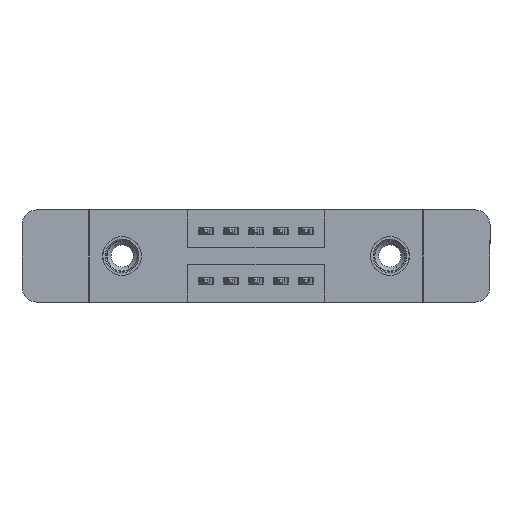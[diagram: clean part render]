
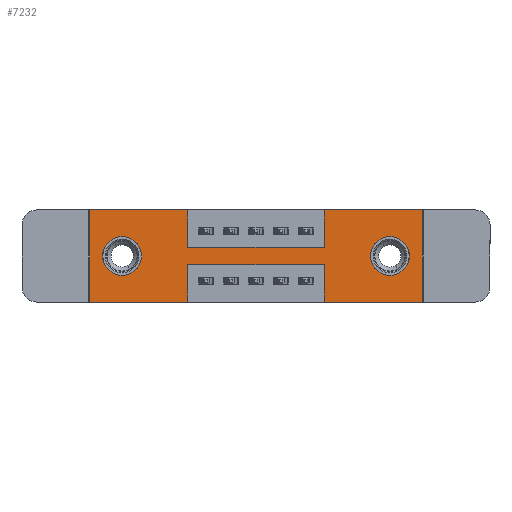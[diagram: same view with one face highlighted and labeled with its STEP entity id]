
A CAD part, front view. The second image highlights one B-rep face of the part: STEP entity #7232.
In plain terms, the highlighted planar face has unit normal (0, -1, 0).
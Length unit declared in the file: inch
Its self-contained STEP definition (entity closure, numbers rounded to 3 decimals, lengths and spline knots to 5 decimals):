
#77 = VERTEX_POINT ( 'NONE', #6850 ) ;
#149 = VECTOR ( 'NONE', #7462, 39.37008 ) ;
#326 = EDGE_CURVE ( 'NONE', #3214, #6701, #7001, .T. ) ;
#468 = DIRECTION ( 'NONE',  ( 0., -1., 0. ) ) ;
#501 = ORIENTED_EDGE ( 'NONE', *, *, #8408, .F. ) ;
#829 = EDGE_LOOP ( 'NONE', ( #4135, #11269 ) ) ;
#876 = DIRECTION ( 'NONE',  ( 0., 0., -1. ) ) ;
#897 = VECTOR ( 'NONE', #2750, 39.37008 ) ;
#1196 = VERTEX_POINT ( 'NONE', #5512 ) ;
#1234 = DIRECTION ( 'NONE',  ( 0., 1., 0. ) ) ;
#1258 = VERTEX_POINT ( 'NONE', #2331 ) ;
#1437 = CARTESIAN_POINT ( 'NONE',  ( 0., 0., -0.37 ) ) ;
#1601 = CARTESIAN_POINT ( 'NONE',  ( 0.13, 0., -0.185 ) ) ;
#1706 = FACE_OUTER_BOUND ( 'NONE', #3340, .T. ) ;
#1759 = DIRECTION ( 'NONE',  ( 0., 0., 1. ) ) ;
#1939 = EDGE_CURVE ( 'NONE', #1196, #9903, #5960, .T. ) ;
#2300 = CIRCLE ( 'NONE', #10257, 0.078 ) ;
#2305 = VERTEX_POINT ( 'NONE', #12155 ) ;
#2312 = CARTESIAN_POINT ( 'NONE',  ( 0.9425, 0., 0. ) ) ;
#2331 = CARTESIAN_POINT ( 'NONE',  ( 0.9425, 0., -0.37 ) ) ;
#2378 = FACE_BOUND ( 'NONE', #8238, .T. ) ;
#2586 = LINE ( 'NONE', #11215, #7533 ) ;
#2589 = CARTESIAN_POINT ( 'NONE',  ( 0., 0., -0.37 ) ) ;
#2598 = ORIENTED_EDGE ( 'NONE', *, *, #13503, .T. ) ;
#2750 = DIRECTION ( 'NONE',  ( 0., 0., -1. ) ) ;
#2804 = LINE ( 'NONE', #5063, #12337 ) ;
#3098 = DIRECTION ( 'NONE',  ( 1., 0., 0. ) ) ;
#3123 = CARTESIAN_POINT ( 'NONE',  ( 0., 0., -0.37 ) ) ;
#3214 = VERTEX_POINT ( 'NONE', #5494 ) ;
#3245 = CARTESIAN_POINT ( 'NONE',  ( 0., 0., 0. ) ) ;
#3257 = AXIS2_PLACEMENT_3D ( 'NONE', #12793, #12705, #6211 ) ;
#3306 = CARTESIAN_POINT ( 'NONE',  ( 1.205, 0., -0.107 ) ) ;
#3326 = VERTEX_POINT ( 'NONE', #8936 ) ;
#3340 = EDGE_LOOP ( 'NONE', ( #4166, #6298, #8539, #12453, #501, #4323, #7828, #5937, #9986, #5646, #8807, #5142 ) ) ;
#3584 = CARTESIAN_POINT ( 'NONE',  ( 0.9425, 0., -0.37 ) ) ;
#3618 = DIRECTION ( 'NONE',  ( 0., 0., -1. ) ) ;
#3710 = PLANE ( 'NONE',  #12693 ) ;
#3730 = CARTESIAN_POINT ( 'NONE',  ( 0.3925, 0., 0. ) ) ;
#3761 = EDGE_CURVE ( 'NONE', #3326, #12559, #2804, .T. ) ;
#3765 = DIRECTION ( 'NONE',  ( 0., 0., -1. ) ) ;
#3780 = LINE ( 'NONE', #6078, #897 ) ;
#3828 = EDGE_CURVE ( 'NONE', #6957, #2305, #9425, .T. ) ;
#4032 = VERTEX_POINT ( 'NONE', #4466 ) ;
#4135 = ORIENTED_EDGE ( 'NONE', *, *, #3828, .T. ) ;
#4166 = ORIENTED_EDGE ( 'NONE', *, *, #5066, .F. ) ;
#4209 = EDGE_CURVE ( 'NONE', #13288, #11241, #8897, .T. ) ;
#4323 = ORIENTED_EDGE ( 'NONE', *, *, #326, .F. ) ;
#4449 = CARTESIAN_POINT ( 'NONE',  ( 0.13, 0., -0.107 ) ) ;
#4466 = CARTESIAN_POINT ( 'NONE',  ( 0.3925, 0., -0.15 ) ) ;
#4483 = EDGE_CURVE ( 'NONE', #6634, #6899, #14109, .T. ) ;
#4513 = CARTESIAN_POINT ( 'NONE',  ( 0., 0., 0. ) ) ;
#4655 = LINE ( 'NONE', #3730, #5844 ) ;
#4662 = DIRECTION ( 'NONE',  ( 0., 0., 1. ) ) ;
#4938 = LINE ( 'NONE', #2312, #9140 ) ;
#4954 = LINE ( 'NONE', #3123, #149 ) ;
#5063 = CARTESIAN_POINT ( 'NONE',  ( 0.3925, 0., -0.22 ) ) ;
#5066 = EDGE_CURVE ( 'NONE', #12559, #13288, #3780, .T. ) ;
#5142 = ORIENTED_EDGE ( 'NONE', *, *, #4209, .F. ) ;
#5155 = VECTOR ( 'NONE', #6878, 39.37008 ) ;
#5494 = CARTESIAN_POINT ( 'NONE',  ( 0.9425, 0., 0. ) ) ;
#5512 = CARTESIAN_POINT ( 'NONE',  ( 1.205, 0., -0.263 ) ) ;
#5526 = CARTESIAN_POINT ( 'NONE',  ( 0., 0., 0. ) ) ;
#5646 = ORIENTED_EDGE ( 'NONE', *, *, #4483, .F. ) ;
#5674 = DIRECTION ( 'NONE',  ( 0., 0., 1. ) ) ;
#5718 = EDGE_CURVE ( 'NONE', #6899, #4032, #4655, .T. ) ;
#5844 = VECTOR ( 'NONE', #876, 39.37008 ) ;
#5937 = ORIENTED_EDGE ( 'NONE', *, *, #6032, .F. ) ;
#5960 = CIRCLE ( 'NONE', #3257, 0.078 ) ;
#6032 = EDGE_CURVE ( 'NONE', #4032, #77, #2586, .T. ) ;
#6078 = CARTESIAN_POINT ( 'NONE',  ( 0.3925, 0., -0.37 ) ) ;
#6211 = DIRECTION ( 'NONE',  ( 0., 0., -1. ) ) ;
#6298 = ORIENTED_EDGE ( 'NONE', *, *, #3761, .F. ) ;
#6305 = CARTESIAN_POINT ( 'NONE',  ( 1.335, 0., -0.37 ) ) ;
#6488 = CARTESIAN_POINT ( 'NONE',  ( 0., 0., 0. ) ) ;
#6634 = VERTEX_POINT ( 'NONE', #4513 ) ;
#6701 = VERTEX_POINT ( 'NONE', #9214 ) ;
#6850 = CARTESIAN_POINT ( 'NONE',  ( 0.9425, 0., -0.15 ) ) ;
#6862 = DIRECTION ( 'NONE',  ( 0., 1., 0. ) ) ;
#6878 = DIRECTION ( 'NONE',  ( 0., 0., 1. ) ) ;
#6899 = VERTEX_POINT ( 'NONE', #10022 ) ;
#6928 = EDGE_CURVE ( 'NONE', #1258, #3326, #7993, .T. ) ;
#6933 = DIRECTION ( 'NONE',  ( 0., 1., 0. ) ) ;
#6957 = VERTEX_POINT ( 'NONE', #4449 ) ;
#7001 = LINE ( 'NONE', #6488, #12428 ) ;
#7232 = ADVANCED_FACE ( 'NONE', ( #2378, #13116, #1706 ), #3710, .T. ) ;
#7245 = DIRECTION ( 'NONE',  ( -1., 0., 0. ) ) ;
#7459 = EDGE_CURVE ( 'NONE', #9203, #1258, #4954, .T. ) ;
#7462 = DIRECTION ( 'NONE',  ( -1., 0., 0. ) ) ;
#7533 = VECTOR ( 'NONE', #9066, 39.37008 ) ;
#7828 = ORIENTED_EDGE ( 'NONE', *, *, #7891, .F. ) ;
#7891 = EDGE_CURVE ( 'NONE', #77, #3214, #4938, .T. ) ;
#7902 = CARTESIAN_POINT ( 'NONE',  ( 1.335, 0., 0. ) ) ;
#7993 = LINE ( 'NONE', #3584, #5155 ) ;
#8165 = CARTESIAN_POINT ( 'NONE',  ( 0.3925, 0., -0.22 ) ) ;
#8202 = EDGE_CURVE ( 'NONE', #11241, #6634, #10683, .T. ) ;
#8215 = CARTESIAN_POINT ( 'NONE',  ( 0., 0., -0.37 ) ) ;
#8238 = EDGE_LOOP ( 'NONE', ( #2598, #11812 ) ) ;
#8408 = EDGE_CURVE ( 'NONE', #6701, #9203, #11704, .T. ) ;
#8441 = AXIS2_PLACEMENT_3D ( 'NONE', #12156, #1234, #11009 ) ;
#8539 = ORIENTED_EDGE ( 'NONE', *, *, #6928, .F. ) ;
#8807 = ORIENTED_EDGE ( 'NONE', *, *, #8202, .F. ) ;
#8897 = LINE ( 'NONE', #8215, #10082 ) ;
#8936 = CARTESIAN_POINT ( 'NONE',  ( 0.9425, 0., -0.22 ) ) ;
#9066 = DIRECTION ( 'NONE',  ( 1., 0., 0. ) ) ;
#9140 = VECTOR ( 'NONE', #5674, 39.37008 ) ;
#9203 = VERTEX_POINT ( 'NONE', #6305 ) ;
#9214 = CARTESIAN_POINT ( 'NONE',  ( 1.335, 0., 0. ) ) ;
#9274 = DIRECTION ( 'NONE',  ( -1., 0., 0. ) ) ;
#9425 = CIRCLE ( 'NONE', #11366, 0.078 ) ;
#9903 = VERTEX_POINT ( 'NONE', #3306 ) ;
#9986 = ORIENTED_EDGE ( 'NONE', *, *, #5718, .F. ) ;
#10022 = CARTESIAN_POINT ( 'NONE',  ( 0.3925, 0., 0. ) ) ;
#10082 = VECTOR ( 'NONE', #7245, 39.37008 ) ;
#10257 = AXIS2_PLACEMENT_3D ( 'NONE', #1601, #6933, #4662 ) ;
#10312 = VECTOR ( 'NONE', #3098, 39.37008 ) ;
#10516 = VECTOR ( 'NONE', #13121, 39.37008 ) ;
#10683 = LINE ( 'NONE', #5526, #10516 ) ;
#10812 = DIRECTION ( 'NONE',  ( 1., 0., 0. ) ) ;
#11009 = DIRECTION ( 'NONE',  ( 0., 0., -1. ) ) ;
#11215 = CARTESIAN_POINT ( 'NONE',  ( 0.3925, 0., -0.15 ) ) ;
#11241 = VERTEX_POINT ( 'NONE', #2589 ) ;
#11269 = ORIENTED_EDGE ( 'NONE', *, *, #14064, .T. ) ;
#11366 = AXIS2_PLACEMENT_3D ( 'NONE', #13342, #6862, #1759 ) ;
#11704 = LINE ( 'NONE', #7902, #13422 ) ;
#11792 = CARTESIAN_POINT ( 'NONE',  ( 0.3925, 0., -0.37 ) ) ;
#11812 = ORIENTED_EDGE ( 'NONE', *, *, #1939, .T. ) ;
#11831 = CIRCLE ( 'NONE', #8441, 0.078 ) ;
#12155 = CARTESIAN_POINT ( 'NONE',  ( 0.13, 0., -0.263 ) ) ;
#12156 = CARTESIAN_POINT ( 'NONE',  ( 1.205, 0., -0.185 ) ) ;
#12337 = VECTOR ( 'NONE', #9274, 39.37008 ) ;
#12428 = VECTOR ( 'NONE', #10812, 39.37008 ) ;
#12453 = ORIENTED_EDGE ( 'NONE', *, *, #7459, .F. ) ;
#12559 = VERTEX_POINT ( 'NONE', #8165 ) ;
#12693 = AXIS2_PLACEMENT_3D ( 'NONE', #1437, #468, #3618 ) ;
#12705 = DIRECTION ( 'NONE',  ( 0., 1., 0. ) ) ;
#12793 = CARTESIAN_POINT ( 'NONE',  ( 1.205, 0., -0.185 ) ) ;
#13116 = FACE_BOUND ( 'NONE', #829, .T. ) ;
#13121 = DIRECTION ( 'NONE',  ( 0., 0., 1. ) ) ;
#13288 = VERTEX_POINT ( 'NONE', #11792 ) ;
#13342 = CARTESIAN_POINT ( 'NONE',  ( 0.13, 0., -0.185 ) ) ;
#13422 = VECTOR ( 'NONE', #3765, 39.37008 ) ;
#13503 = EDGE_CURVE ( 'NONE', #9903, #1196, #11831, .T. ) ;
#14064 = EDGE_CURVE ( 'NONE', #2305, #6957, #2300, .T. ) ;
#14109 = LINE ( 'NONE', #3245, #10312 ) ;
